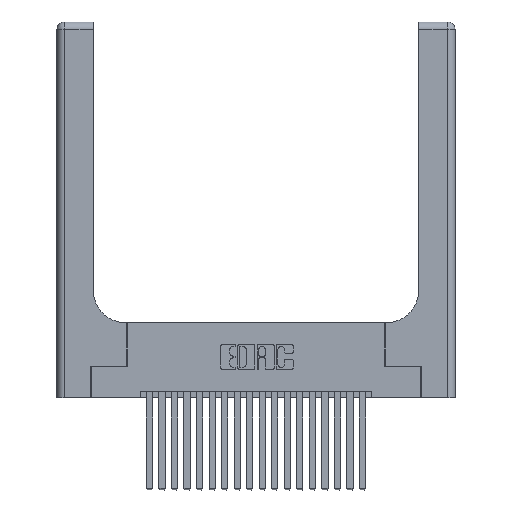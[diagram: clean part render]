
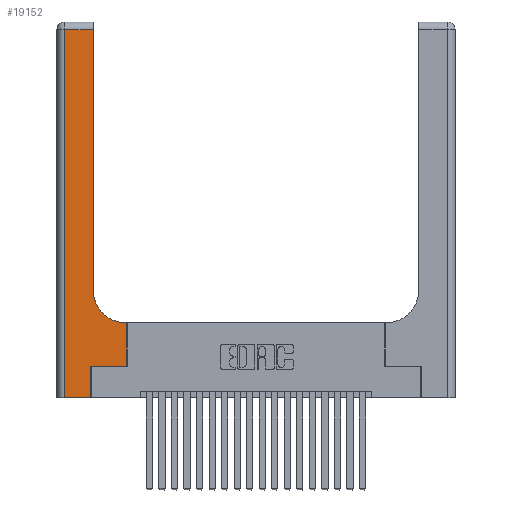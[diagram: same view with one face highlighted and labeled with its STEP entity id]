
A CAD part, top view. The second image highlights one B-rep face of the part: STEP entity #19152.
In plain terms, the highlighted planar face has unit normal (0, 0, 1).
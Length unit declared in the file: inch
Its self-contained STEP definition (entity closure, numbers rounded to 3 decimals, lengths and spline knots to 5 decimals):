
#490 = EDGE_CURVE ( 'NONE', #15788, #15045, #17290, .T. ) ;
#582 = ORIENTED_EDGE ( 'NONE', *, *, #5284, .T. ) ;
#895 = DIRECTION ( 'NONE',  ( -1., 0., 0. ) ) ;
#1024 = DIRECTION ( 'NONE',  ( 1., 0., 0. ) ) ;
#1452 = DIRECTION ( 'NONE',  ( 1., 0., 0. ) ) ;
#1581 = ORIENTED_EDGE ( 'NONE', *, *, #7356, .T. ) ;
#1750 = CARTESIAN_POINT ( 'NONE',  ( 0.2915, 2.94, 0.37 ) ) ;
#1976 = LINE ( 'NONE', #20004, #16345 ) ;
#1989 = CARTESIAN_POINT ( 'NONE',  ( 0.06, 0., 0.37 ) ) ;
#2591 = CARTESIAN_POINT ( 'NONE',  ( 0., 3., 0.37 ) ) ;
#2727 = CARTESIAN_POINT ( 'NONE',  ( 0.5585, 0.6, 0.37 ) ) ;
#3633 = VERTEX_POINT ( 'NONE', #7885 ) ;
#4048 = VECTOR ( 'NONE', #9179, 39.37008 ) ;
#4147 = VECTOR ( 'NONE', #18121, 39.37008 ) ;
#4318 = VERTEX_POINT ( 'NONE', #16665 ) ;
#4710 = DIRECTION ( 'NONE',  ( -1., 0., 0. ) ) ;
#5243 = VECTOR ( 'NONE', #5762, 39.37008 ) ;
#5284 = EDGE_CURVE ( 'NONE', #4318, #10709, #10359, .T. ) ;
#5351 = EDGE_CURVE ( 'NONE', #10709, #13078, #8764, .T. ) ;
#5403 = VECTOR ( 'NONE', #4710, 39.37008 ) ;
#5762 = DIRECTION ( 'NONE',  ( 1., 0., 0. ) ) ;
#6205 = LINE ( 'NONE', #12310, #8743 ) ;
#6288 = CARTESIAN_POINT ( 'NONE',  ( 0.269, 0., 0.37 ) ) ;
#6519 = ORIENTED_EDGE ( 'NONE', *, *, #13099, .T. ) ;
#7356 = EDGE_CURVE ( 'NONE', #21079, #4318, #12753, .T. ) ;
#7885 = CARTESIAN_POINT ( 'NONE',  ( 0.5415, 0.6, 0.37 ) ) ;
#8234 = VECTOR ( 'NONE', #17989, 39.37008 ) ;
#8420 = VERTEX_POINT ( 'NONE', #1750 ) ;
#8493 = ORIENTED_EDGE ( 'NONE', *, *, #10104, .T. ) ;
#8496 = CIRCLE ( 'NONE', #11573, 0.25 ) ;
#8743 = VECTOR ( 'NONE', #8889, 39.37008 ) ;
#8764 = LINE ( 'NONE', #9448, #4147 ) ;
#8889 = DIRECTION ( 'NONE',  ( 0., 1., 0. ) ) ;
#9129 = ORIENTED_EDGE ( 'NONE', *, *, #13147, .T. ) ;
#9152 = CARTESIAN_POINT ( 'NONE',  ( 0.06, 3., 0.37 ) ) ;
#9179 = DIRECTION ( 'NONE',  ( 0., -1., 0. ) ) ;
#9448 = CARTESIAN_POINT ( 'NONE',  ( 0.5585, 0.25, 0.37 ) ) ;
#9597 = LINE ( 'NONE', #10005, #18791 ) ;
#10005 = CARTESIAN_POINT ( 'NONE',  ( 0., 2.94, 0.37 ) ) ;
#10014 = LINE ( 'NONE', #13300, #5403 ) ;
#10104 = EDGE_CURVE ( 'NONE', #13078, #3633, #10014, .T. ) ;
#10359 = LINE ( 'NONE', #19557, #5243 ) ;
#10709 = VERTEX_POINT ( 'NONE', #18281 ) ;
#11266 = DIRECTION ( 'NONE',  ( 0., 0., -1. ) ) ;
#11294 = CARTESIAN_POINT ( 'NONE',  ( 0.2915, 0.85, 0.37 ) ) ;
#11573 = AXIS2_PLACEMENT_3D ( 'NONE', #22096, #11812, #1452 ) ;
#11812 = DIRECTION ( 'NONE',  ( 0., 0., -1. ) ) ;
#12118 = EDGE_LOOP ( 'NONE', ( #14578, #9129, #18712, #6519, #1581, #582, #16813, #8493, #18615 ) ) ;
#12310 = CARTESIAN_POINT ( 'NONE',  ( 0.2915, 3., 0.37 ) ) ;
#12753 = LINE ( 'NONE', #12760, #8234 ) ;
#12760 = CARTESIAN_POINT ( 'NONE',  ( 0.269, 0., 0.37 ) ) ;
#13078 = VERTEX_POINT ( 'NONE', #2727 ) ;
#13099 = EDGE_CURVE ( 'NONE', #15045, #21079, #1976, .T. ) ;
#13147 = EDGE_CURVE ( 'NONE', #8420, #15788, #9597, .T. ) ;
#13300 = CARTESIAN_POINT ( 'NONE',  ( 0.2915, 0.6, 0.37 ) ) ;
#13895 = EDGE_CURVE ( 'NONE', #3633, #17088, #8496, .T. ) ;
#14126 = EDGE_CURVE ( 'NONE', #17088, #8420, #6205, .T. ) ;
#14578 = ORIENTED_EDGE ( 'NONE', *, *, #14126, .T. ) ;
#15045 = VERTEX_POINT ( 'NONE', #1989 ) ;
#15788 = VERTEX_POINT ( 'NONE', #19744 ) ;
#16345 = VECTOR ( 'NONE', #1024, 39.37008 ) ;
#16436 = PLANE ( 'NONE',  #21272 ) ;
#16665 = CARTESIAN_POINT ( 'NONE',  ( 0.269, 0.25, 0.37 ) ) ;
#16813 = ORIENTED_EDGE ( 'NONE', *, *, #5351, .T. ) ;
#17088 = VERTEX_POINT ( 'NONE', #11294 ) ;
#17290 = LINE ( 'NONE', #9152, #4048 ) ;
#17989 = DIRECTION ( 'NONE',  ( 0., 1., 0. ) ) ;
#18121 = DIRECTION ( 'NONE',  ( 0., 1., 0. ) ) ;
#18281 = CARTESIAN_POINT ( 'NONE',  ( 0.5585, 0.25, 0.37 ) ) ;
#18615 = ORIENTED_EDGE ( 'NONE', *, *, #13895, .T. ) ;
#18712 = ORIENTED_EDGE ( 'NONE', *, *, #490, .T. ) ;
#18791 = VECTOR ( 'NONE', #21972, 39.37008 ) ;
#19152 = ADVANCED_FACE ( 'NONE', ( #19358 ), #16436, .F. ) ;
#19358 = FACE_OUTER_BOUND ( 'NONE', #12118, .T. ) ;
#19557 = CARTESIAN_POINT ( 'NONE',  ( 0.269, 0.25, 0.37 ) ) ;
#19744 = CARTESIAN_POINT ( 'NONE',  ( 0.06, 2.94, 0.37 ) ) ;
#20004 = CARTESIAN_POINT ( 'NONE',  ( 0., 0., 0.37 ) ) ;
#21079 = VERTEX_POINT ( 'NONE', #6288 ) ;
#21272 = AXIS2_PLACEMENT_3D ( 'NONE', #2591, #11266, #895 ) ;
#21972 = DIRECTION ( 'NONE',  ( -1., 0., 0. ) ) ;
#22096 = CARTESIAN_POINT ( 'NONE',  ( 0.5415, 0.85, 0.37 ) ) ;
